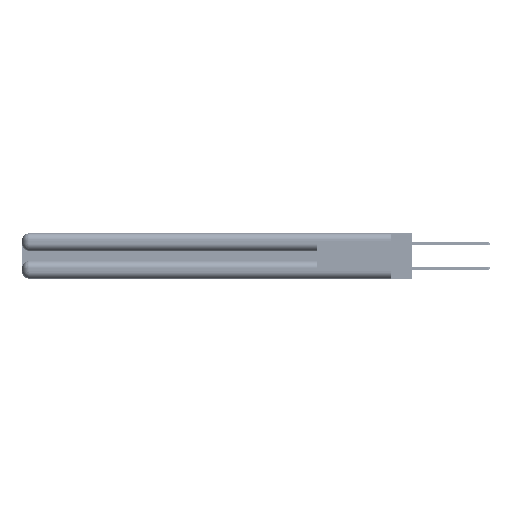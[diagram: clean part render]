
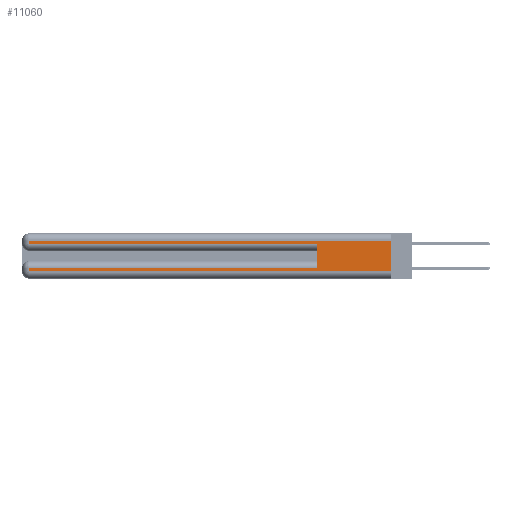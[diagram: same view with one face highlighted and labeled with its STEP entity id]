
A CAD part, left-side view. The second image highlights one B-rep face of the part: STEP entity #11060.
In plain terms, the highlighted planar face has unit normal (-1, 0, 0).
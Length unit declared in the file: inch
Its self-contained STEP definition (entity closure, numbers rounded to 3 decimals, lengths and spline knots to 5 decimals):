
#944 = CARTESIAN_POINT ( 'NONE',  ( 0., 2.94, 0.06 ) ) ;
#997 = CARTESIAN_POINT ( 'NONE',  ( 0., 0., 0.285 ) ) ;
#1190 = DIRECTION ( 'NONE',  ( 0., -1., 0. ) ) ;
#1196 = EDGE_CURVE ( 'NONE', #22128, #40133, #52392, .T. ) ;
#1555 = LINE ( 'NONE', #5128, #14226 ) ;
#2062 = EDGE_CURVE ( 'NONE', #34917, #11222, #1555, .T. ) ;
#2072 = LINE ( 'NONE', #20265, #45580 ) ;
#2483 = ORIENTED_EDGE ( 'NONE', *, *, #40849, .T. ) ;
#3136 = EDGE_CURVE ( 'NONE', #41874, #36862, #2072, .T. ) ;
#3519 = CARTESIAN_POINT ( 'NONE',  ( 0., 2.94, 0.37 ) ) ;
#3747 = ORIENTED_EDGE ( 'NONE', *, *, #39468, .F. ) ;
#5128 = CARTESIAN_POINT ( 'NONE',  ( 0., 0., 0.31 ) ) ;
#5518 = VERTEX_POINT ( 'NONE', #38012 ) ;
#7852 = DIRECTION ( 'NONE',  ( 0., 0., -1. ) ) ;
#9306 = LINE ( 'NONE', #54288, #41517 ) ;
#9618 = VECTOR ( 'NONE', #7852, 39.37008 ) ;
#9622 = VECTOR ( 'NONE', #49845, 39.37008 ) ;
#11060 = ADVANCED_FACE ( 'NONE', ( #26627 ), #16716, .F. ) ;
#11222 = VERTEX_POINT ( 'NONE', #13338 ) ;
#11425 = CARTESIAN_POINT ( 'NONE',  ( 0., 2.94, 0.085 ) ) ;
#13338 = CARTESIAN_POINT ( 'NONE',  ( 0., 2.94, 0.31 ) ) ;
#14226 = VECTOR ( 'NONE', #30442, 39.37008 ) ;
#16307 = CARTESIAN_POINT ( 'NONE',  ( 0., 0., 0.37 ) ) ;
#16716 = PLANE ( 'NONE',  #18341 ) ;
#18245 = LINE ( 'NONE', #16307, #9622 ) ;
#18341 = AXIS2_PLACEMENT_3D ( 'NONE', #25003, #46020, #20958 ) ;
#18979 = VECTOR ( 'NONE', #1190, 39.37008 ) ;
#20265 = CARTESIAN_POINT ( 'NONE',  ( 0., 0., 0.085 ) ) ;
#20958 = DIRECTION ( 'NONE',  ( 0., 0., -1. ) ) ;
#22128 = VERTEX_POINT ( 'NONE', #54040 ) ;
#22341 = CARTESIAN_POINT ( 'NONE',  ( 0., 0.6, 0.145 ) ) ;
#22663 = CARTESIAN_POINT ( 'NONE',  ( 0., 0.6, 0.285 ) ) ;
#22926 = ORIENTED_EDGE ( 'NONE', *, *, #35795, .T. ) ;
#23560 = EDGE_LOOP ( 'NONE', ( #25739, #49744, #37996, #45585, #3747, #28353, #22926, #2483 ) ) ;
#25003 = CARTESIAN_POINT ( 'NONE',  ( 0., 0., 0.37 ) ) ;
#25739 = ORIENTED_EDGE ( 'NONE', *, *, #26095, .F. ) ;
#26095 = EDGE_CURVE ( 'NONE', #34917, #5518, #18245, .T. ) ;
#26559 = DIRECTION ( 'NONE',  ( 0., 0., 1. ) ) ;
#26627 = FACE_OUTER_BOUND ( 'NONE', #23560, .T. ) ;
#28353 = ORIENTED_EDGE ( 'NONE', *, *, #3136, .T. ) ;
#28923 = VERTEX_POINT ( 'NONE', #944 ) ;
#29228 = DIRECTION ( 'NONE',  ( 0., 0., -1. ) ) ;
#30442 = DIRECTION ( 'NONE',  ( 0., 1., 0. ) ) ;
#33809 = VECTOR ( 'NONE', #39392, 39.37008 ) ;
#34917 = VERTEX_POINT ( 'NONE', #37705 ) ;
#35114 = LINE ( 'NONE', #51870, #33809 ) ;
#35795 = EDGE_CURVE ( 'NONE', #36862, #28923, #43137, .T. ) ;
#36862 = VERTEX_POINT ( 'NONE', #11425 ) ;
#37457 = VECTOR ( 'NONE', #26559, 39.37008 ) ;
#37705 = CARTESIAN_POINT ( 'NONE',  ( 0., 0., 0.31 ) ) ;
#37996 = ORIENTED_EDGE ( 'NONE', *, *, #38540, .T. ) ;
#38012 = CARTESIAN_POINT ( 'NONE',  ( 0., 0., 0.06 ) ) ;
#38540 = EDGE_CURVE ( 'NONE', #11222, #22128, #9306, .T. ) ;
#39392 = DIRECTION ( 'NONE',  ( 0., -1., 0. ) ) ;
#39468 = EDGE_CURVE ( 'NONE', #41874, #40133, #48629, .T. ) ;
#40133 = VERTEX_POINT ( 'NONE', #22663 ) ;
#40849 = EDGE_CURVE ( 'NONE', #28923, #5518, #35114, .T. ) ;
#41517 = VECTOR ( 'NONE', #29228, 39.37008 ) ;
#41874 = VERTEX_POINT ( 'NONE', #44723 ) ;
#43137 = LINE ( 'NONE', #3519, #9618 ) ;
#44723 = CARTESIAN_POINT ( 'NONE',  ( 0., 0.6, 0.085 ) ) ;
#45580 = VECTOR ( 'NONE', #49548, 39.37008 ) ;
#45585 = ORIENTED_EDGE ( 'NONE', *, *, #1196, .T. ) ;
#46020 = DIRECTION ( 'NONE',  ( 1., 0., 0. ) ) ;
#48629 = LINE ( 'NONE', #22341, #37457 ) ;
#49548 = DIRECTION ( 'NONE',  ( 0., 1., 0. ) ) ;
#49744 = ORIENTED_EDGE ( 'NONE', *, *, #2062, .T. ) ;
#49845 = DIRECTION ( 'NONE',  ( 0., 0., -1. ) ) ;
#51870 = CARTESIAN_POINT ( 'NONE',  ( 0., 0., 0.06 ) ) ;
#52392 = LINE ( 'NONE', #997, #18979 ) ;
#54040 = CARTESIAN_POINT ( 'NONE',  ( 0., 2.94, 0.285 ) ) ;
#54288 = CARTESIAN_POINT ( 'NONE',  ( 0., 2.94, 0.37 ) ) ;
